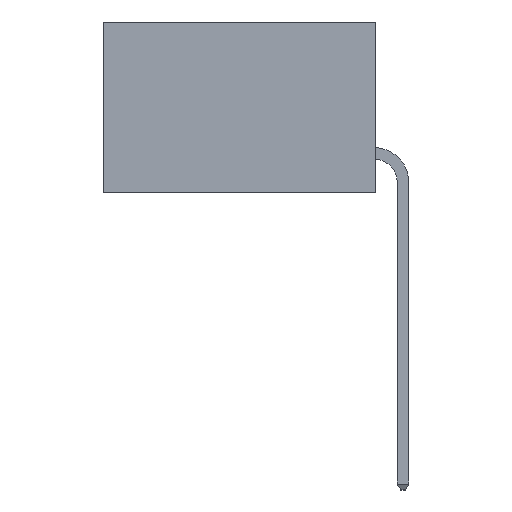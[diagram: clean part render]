
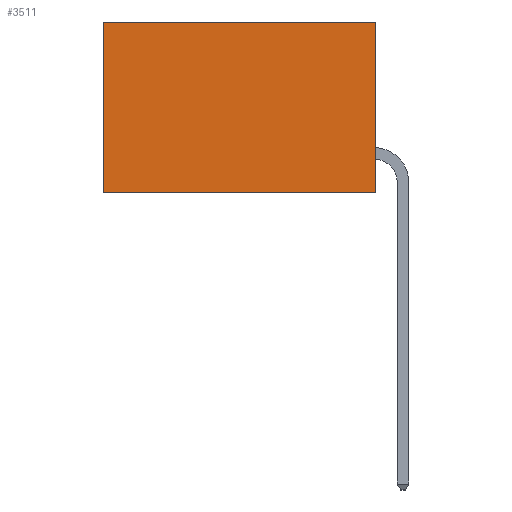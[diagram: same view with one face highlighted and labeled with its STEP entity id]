
A CAD part, left-side view. The second image highlights one B-rep face of the part: STEP entity #3511.
In plain terms, the highlighted planar face has unit normal (-1, 0, 0).
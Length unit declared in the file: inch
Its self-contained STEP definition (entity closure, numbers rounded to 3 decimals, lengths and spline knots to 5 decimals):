
#98 = VERTEX_POINT ( 'NONE', #9452 ) ;
#292 = VECTOR ( 'NONE', #14242, 39.37008 ) ;
#442 = CARTESIAN_POINT ( 'NONE',  ( 0.277, 0., -0.37 ) ) ;
#646 = ORIENTED_EDGE ( 'NONE', *, *, #11034, .F. ) ;
#1209 = ORIENTED_EDGE ( 'NONE', *, *, #6024, .T. ) ;
#2610 = CARTESIAN_POINT ( 'NONE',  ( 0.277, 0., -0.37 ) ) ;
#3511 = ADVANCED_FACE ( 'NONE', ( #12765 ), #12653, .F. ) ;
#3525 = CARTESIAN_POINT ( 'NONE',  ( 0.277, 0.59, -0.37 ) ) ;
#3533 = LINE ( 'NONE', #14254, #292 ) ;
#3628 = LINE ( 'NONE', #442, #7883 ) ;
#3922 = DIRECTION ( 'NONE',  ( 0., 0., -1. ) ) ;
#4159 = CARTESIAN_POINT ( 'NONE',  ( 0.277, 0., -0.37 ) ) ;
#5510 = VERTEX_POINT ( 'NONE', #3525 ) ;
#6024 = EDGE_CURVE ( 'NONE', #98, #16893, #3533, .T. ) ;
#7386 = EDGE_CURVE ( 'NONE', #12024, #5510, #16614, .T. ) ;
#7624 = EDGE_LOOP ( 'NONE', ( #19352, #8425, #646, #1209 ) ) ;
#7721 = CARTESIAN_POINT ( 'NONE',  ( 0.277, 0.59, 0. ) ) ;
#7883 = VECTOR ( 'NONE', #11509, 39.37008 ) ;
#8425 = ORIENTED_EDGE ( 'NONE', *, *, #7386, .F. ) ;
#9170 = AXIS2_PLACEMENT_3D ( 'NONE', #4159, #12783, #11692 ) ;
#9452 = CARTESIAN_POINT ( 'NONE',  ( 0.277, 0., 0. ) ) ;
#10221 = CARTESIAN_POINT ( 'NONE',  ( 0.277, 0.59, -0.37 ) ) ;
#10554 = LINE ( 'NONE', #10221, #13174 ) ;
#11034 = EDGE_CURVE ( 'NONE', #98, #12024, #3628, .T. ) ;
#11160 = EDGE_CURVE ( 'NONE', #16893, #5510, #10554, .T. ) ;
#11509 = DIRECTION ( 'NONE',  ( 0., 0., -1. ) ) ;
#11692 = DIRECTION ( 'NONE',  ( 0., 0., -1. ) ) ;
#12024 = VERTEX_POINT ( 'NONE', #2610 ) ;
#12653 = PLANE ( 'NONE',  #9170 ) ;
#12765 = FACE_OUTER_BOUND ( 'NONE', #7624, .T. ) ;
#12783 = DIRECTION ( 'NONE',  ( 1., 0., 0. ) ) ;
#13174 = VECTOR ( 'NONE', #3922, 39.37008 ) ;
#14242 = DIRECTION ( 'NONE',  ( 0., 1., 0. ) ) ;
#14254 = CARTESIAN_POINT ( 'NONE',  ( 0.277, 0., 0. ) ) ;
#16085 = CARTESIAN_POINT ( 'NONE',  ( 0.277, 0., -0.37 ) ) ;
#16154 = VECTOR ( 'NONE', #16264, 39.37008 ) ;
#16264 = DIRECTION ( 'NONE',  ( 0., 1., 0. ) ) ;
#16614 = LINE ( 'NONE', #16085, #16154 ) ;
#16893 = VERTEX_POINT ( 'NONE', #7721 ) ;
#19352 = ORIENTED_EDGE ( 'NONE', *, *, #11160, .T. ) ;
